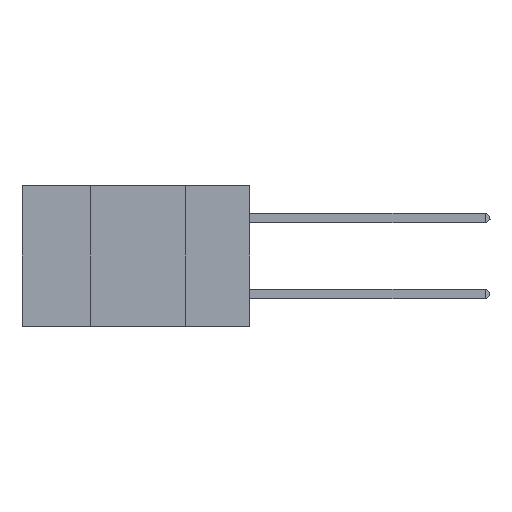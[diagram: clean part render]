
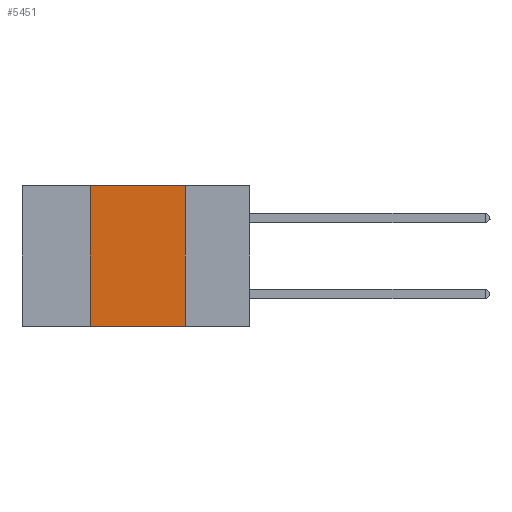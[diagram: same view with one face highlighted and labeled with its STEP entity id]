
A CAD part, left-side view. The second image highlights one B-rep face of the part: STEP entity #5451.
In plain terms, the highlighted planar face has unit normal (-1, 0, 0).
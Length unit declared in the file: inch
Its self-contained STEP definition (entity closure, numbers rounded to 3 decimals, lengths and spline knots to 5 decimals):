
#251 = DIRECTION ( 'NONE',  ( 0., -1., 0. ) ) ;
#558 = CARTESIAN_POINT ( 'NONE',  ( 0., 0.17, 0. ) ) ;
#1930 = EDGE_CURVE ( 'NONE', #8239, #18168, #7089, .T. ) ;
#2452 = ORIENTED_EDGE ( 'NONE', *, *, #19450, .T. ) ;
#3881 = EDGE_LOOP ( 'NONE', ( #29401, #15961, #5696, #2452 ) ) ;
#5130 = CARTESIAN_POINT ( 'NONE',  ( 0., 0.6, -0.37 ) ) ;
#5451 = ADVANCED_FACE ( 'NONE', ( #14506 ), #14959, .F. ) ;
#5696 = ORIENTED_EDGE ( 'NONE', *, *, #1930, .F. ) ;
#6962 = VECTOR ( 'NONE', #18518, 39.37008 ) ;
#7089 = LINE ( 'NONE', #25404, #6962 ) ;
#7541 = DIRECTION ( 'NONE',  ( 0., 0., -1. ) ) ;
#8239 = VERTEX_POINT ( 'NONE', #24555 ) ;
#9771 = VECTOR ( 'NONE', #251, 39.37008 ) ;
#10090 = LINE ( 'NONE', #19717, #23441 ) ;
#11656 = CARTESIAN_POINT ( 'NONE',  ( 0., 0.6, 0. ) ) ;
#12037 = DIRECTION ( 'NONE',  ( 0., -1., 0. ) ) ;
#12743 = CARTESIAN_POINT ( 'NONE',  ( 0., 0.42, 0. ) ) ;
#13496 = VERTEX_POINT ( 'NONE', #27638 ) ;
#13925 = EDGE_CURVE ( 'NONE', #18168, #18532, #28009, .T. ) ;
#14506 = FACE_OUTER_BOUND ( 'NONE', #3881, .T. ) ;
#14959 = PLANE ( 'NONE',  #26283 ) ;
#15961 = ORIENTED_EDGE ( 'NONE', *, *, #13925, .F. ) ;
#16089 = VECTOR ( 'NONE', #12037, 39.37008 ) ;
#16918 = CARTESIAN_POINT ( 'NONE',  ( 0., 0.6, 0. ) ) ;
#18168 = VERTEX_POINT ( 'NONE', #12743 ) ;
#18518 = DIRECTION ( 'NONE',  ( 0., 0., 1. ) ) ;
#18532 = VERTEX_POINT ( 'NONE', #558 ) ;
#19014 = DIRECTION ( 'NONE',  ( 0., 0., -1. ) ) ;
#19450 = EDGE_CURVE ( 'NONE', #8239, #13496, #25696, .T. ) ;
#19717 = CARTESIAN_POINT ( 'NONE',  ( 0., 0.17, 0. ) ) ;
#23441 = VECTOR ( 'NONE', #7541, 39.37008 ) ;
#23616 = EDGE_CURVE ( 'NONE', #18532, #13496, #10090, .T. ) ;
#24106 = DIRECTION ( 'NONE',  ( 1., 0., 0. ) ) ;
#24555 = CARTESIAN_POINT ( 'NONE',  ( 0., 0.42, -0.37 ) ) ;
#25404 = CARTESIAN_POINT ( 'NONE',  ( 0., 0.42, 0. ) ) ;
#25696 = LINE ( 'NONE', #5130, #16089 ) ;
#26283 = AXIS2_PLACEMENT_3D ( 'NONE', #16918, #24106, #19014 ) ;
#27638 = CARTESIAN_POINT ( 'NONE',  ( 0., 0.17, -0.37 ) ) ;
#28009 = LINE ( 'NONE', #11656, #9771 ) ;
#29401 = ORIENTED_EDGE ( 'NONE', *, *, #23616, .F. ) ;
